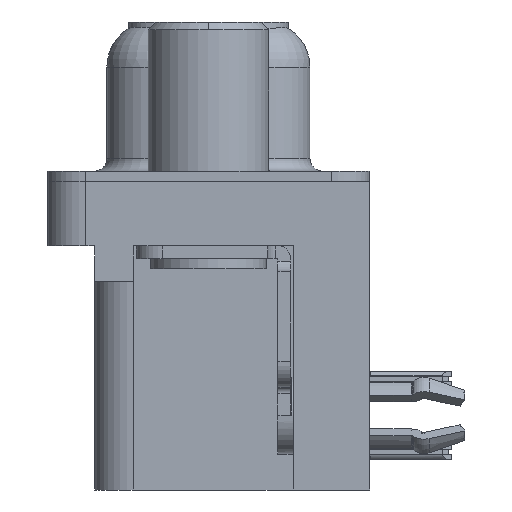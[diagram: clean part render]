
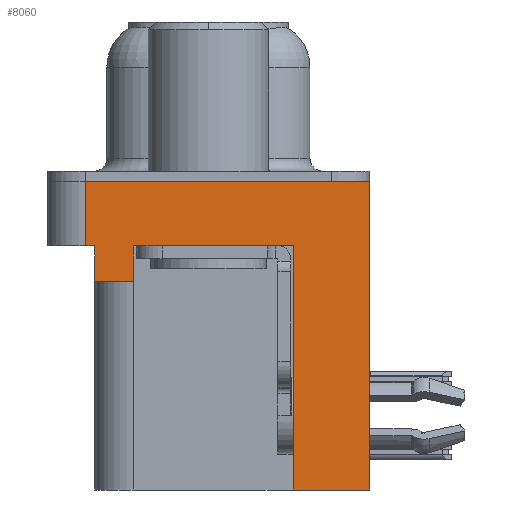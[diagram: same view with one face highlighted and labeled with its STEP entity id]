
A CAD part, left-side view. The second image highlights one B-rep face of the part: STEP entity #8060.
In plain terms, the highlighted planar face has unit normal (-1, 0, 0).
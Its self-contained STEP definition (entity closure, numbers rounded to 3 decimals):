
#18 = CARTESIAN_POINT ( 'NONE',  ( -3., -6.275, 0. ) ) ;
#204 = CARTESIAN_POINT ( 'NONE',  ( -3., -3.295, -12. ) ) ;
#233 = DIRECTION ( 'NONE',  ( -1., 0., 0. ) ) ;
#569 = CARTESIAN_POINT ( 'NONE',  ( -3., -3.295, -12. ) ) ;
#1078 = CARTESIAN_POINT ( 'NONE',  ( -3., 2.895, -3.9 ) ) ;
#1806 = VECTOR ( 'NONE', #23420, 1000. ) ;
#1961 = CARTESIAN_POINT ( 'NONE',  ( -3., 4.775, -2.5 ) ) ;
#2756 = CARTESIAN_POINT ( 'NONE',  ( -3., 4.425, -3.9 ) ) ;
#2762 = VERTEX_POINT ( 'NONE', #25296 ) ;
#2880 = CARTESIAN_POINT ( 'NONE',  ( -3., 4.775, 0. ) ) ;
#3160 = DIRECTION ( 'NONE',  ( 0., 0., 1. ) ) ;
#3224 = EDGE_CURVE ( 'NONE', #24742, #12842, #29145, .T. ) ;
#3459 = ORIENTED_EDGE ( 'NONE', *, *, #3224, .F. ) ;
#4024 = CARTESIAN_POINT ( 'NONE',  ( -3., -6.275, -12. ) ) ;
#4557 = DIRECTION ( 'NONE',  ( 0., 0., 1. ) ) ;
#4788 = CARTESIAN_POINT ( 'NONE',  ( -3., 2.895, -3.9 ) ) ;
#4990 = ORIENTED_EDGE ( 'NONE', *, *, #7673, .T. ) ;
#5591 = FACE_OUTER_BOUND ( 'NONE', #27696, .T. ) ;
#6202 = ORIENTED_EDGE ( 'NONE', *, *, #17268, .F. ) ;
#6391 = DIRECTION ( 'NONE',  ( 0., 0., 1. ) ) ;
#6603 = ORIENTED_EDGE ( 'NONE', *, *, #27426, .T. ) ;
#7425 = LINE ( 'NONE', #18628, #22167 ) ;
#7673 = EDGE_CURVE ( 'NONE', #13181, #8097, #17570, .T. ) ;
#7809 = CARTESIAN_POINT ( 'NONE',  ( -3., -6.275, -2.5 ) ) ;
#8060 = ADVANCED_FACE ( 'NONE', ( #5591 ), #30386, .T. ) ;
#8097 = VERTEX_POINT ( 'NONE', #11093 ) ;
#8626 = LINE ( 'NONE', #569, #1806 ) ;
#9182 = DIRECTION ( 'NONE',  ( 0., -1., 0. ) ) ;
#9493 = CARTESIAN_POINT ( 'NONE',  ( -3., -3.295, -12. ) ) ;
#9501 = VECTOR ( 'NONE', #10332, 1000. ) ;
#10332 = DIRECTION ( 'NONE',  ( 0., -1., 0. ) ) ;
#10499 = ORIENTED_EDGE ( 'NONE', *, *, #31560, .T. ) ;
#10663 = DIRECTION ( 'NONE',  ( 0., 0., 1. ) ) ;
#11093 = CARTESIAN_POINT ( 'NONE',  ( -3., 4.425, -2.5 ) ) ;
#11334 = CARTESIAN_POINT ( 'NONE',  ( -3., 4.425, -3.9 ) ) ;
#12175 = LINE ( 'NONE', #23357, #25803 ) ;
#12842 = VERTEX_POINT ( 'NONE', #11334 ) ;
#13181 = VERTEX_POINT ( 'NONE', #25565 ) ;
#13841 = DIRECTION ( 'NONE',  ( 0., 1., 0. ) ) ;
#14226 = VECTOR ( 'NONE', #19731, 1000. ) ;
#14306 = VERTEX_POINT ( 'NONE', #18 ) ;
#14490 = EDGE_CURVE ( 'NONE', #12842, #8097, #12175, .T. ) ;
#14794 = VERTEX_POINT ( 'NONE', #4024 ) ;
#15071 = CARTESIAN_POINT ( 'NONE',  ( -3., -6.275, -2.5 ) ) ;
#15777 = LINE ( 'NONE', #1078, #20524 ) ;
#16001 = LINE ( 'NONE', #204, #30777 ) ;
#16350 = VECTOR ( 'NONE', #13841, 1000. ) ;
#17268 = EDGE_CURVE ( 'NONE', #13181, #19467, #25290, .T. ) ;
#17570 = LINE ( 'NONE', #21890, #32385 ) ;
#17893 = LINE ( 'NONE', #7809, #9501 ) ;
#18347 = DIRECTION ( 'NONE',  ( 0., 0., 1. ) ) ;
#18628 = CARTESIAN_POINT ( 'NONE',  ( -3., -6.275, 0. ) ) ;
#19390 = EDGE_CURVE ( 'NONE', #31226, #2762, #16001, .T. ) ;
#19467 = VERTEX_POINT ( 'NONE', #2880 ) ;
#19731 = DIRECTION ( 'NONE',  ( 0., 0., 1. ) ) ;
#20524 = VECTOR ( 'NONE', #6391, 1000. ) ;
#21414 = DIRECTION ( 'NONE',  ( 0., -1., 0. ) ) ;
#21890 = CARTESIAN_POINT ( 'NONE',  ( -3., -6.275, -2.5 ) ) ;
#22167 = VECTOR ( 'NONE', #21414, 1000. ) ;
#22860 = ORIENTED_EDGE ( 'NONE', *, *, #24719, .T. ) ;
#23335 = AXIS2_PLACEMENT_3D ( 'NONE', #15071, #233, #10663 ) ;
#23357 = CARTESIAN_POINT ( 'NONE',  ( -3., 4.425, -3.9 ) ) ;
#23420 = DIRECTION ( 'NONE',  ( 0., 1., 0. ) ) ;
#24277 = LINE ( 'NONE', #25232, #14226 ) ;
#24719 = EDGE_CURVE ( 'NONE', #14794, #14306, #24277, .T. ) ;
#24742 = VERTEX_POINT ( 'NONE', #4788 ) ;
#24964 = EDGE_CURVE ( 'NONE', #14794, #31226, #8626, .T. ) ;
#25232 = CARTESIAN_POINT ( 'NONE',  ( -3., -6.275, -2.5 ) ) ;
#25290 = LINE ( 'NONE', #1961, #28863 ) ;
#25296 = CARTESIAN_POINT ( 'NONE',  ( -3., -3.295, -2.5 ) ) ;
#25565 = CARTESIAN_POINT ( 'NONE',  ( -3., 4.775, -2.5 ) ) ;
#25567 = EDGE_CURVE ( 'NONE', #19467, #14306, #7425, .T. ) ;
#25803 = VECTOR ( 'NONE', #3160, 1000. ) ;
#27426 = EDGE_CURVE ( 'NONE', #24742, #28849, #15777, .T. ) ;
#27696 = EDGE_LOOP ( 'NONE', ( #32857, #6202, #4990, #29346, #3459, #6603, #10499, #29230, #29770, #22860 ) ) ;
#28849 = VERTEX_POINT ( 'NONE', #32748 ) ;
#28863 = VECTOR ( 'NONE', #4557, 1000. ) ;
#29145 = LINE ( 'NONE', #2756, #16350 ) ;
#29230 = ORIENTED_EDGE ( 'NONE', *, *, #19390, .F. ) ;
#29346 = ORIENTED_EDGE ( 'NONE', *, *, #14490, .F. ) ;
#29770 = ORIENTED_EDGE ( 'NONE', *, *, #24964, .F. ) ;
#30386 = PLANE ( 'NONE',  #23335 ) ;
#30777 = VECTOR ( 'NONE', #18347, 1000. ) ;
#31226 = VERTEX_POINT ( 'NONE', #9493 ) ;
#31560 = EDGE_CURVE ( 'NONE', #28849, #2762, #17893, .T. ) ;
#32385 = VECTOR ( 'NONE', #9182, 1000. ) ;
#32748 = CARTESIAN_POINT ( 'NONE',  ( -3., 2.895, -2.5 ) ) ;
#32857 = ORIENTED_EDGE ( 'NONE', *, *, #25567, .F. ) ;
